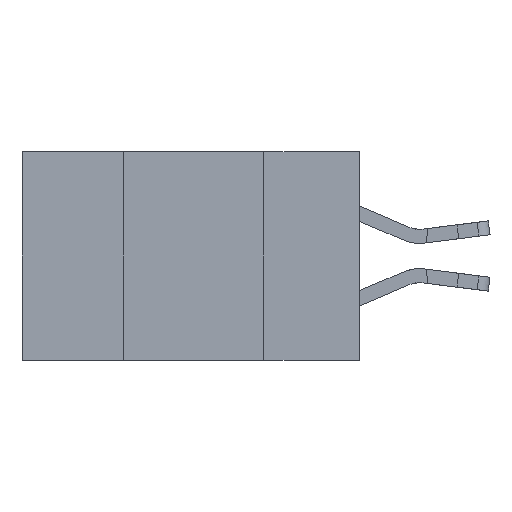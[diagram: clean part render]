
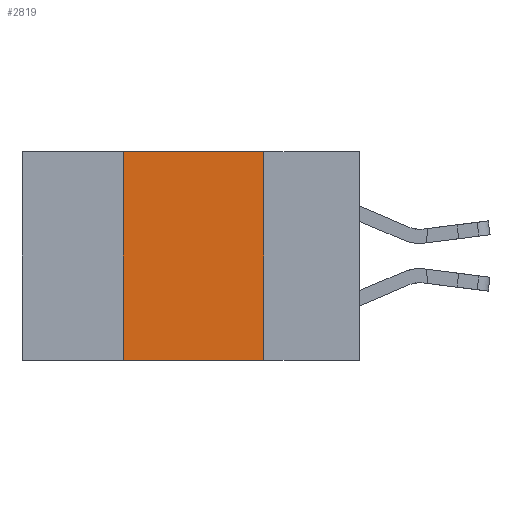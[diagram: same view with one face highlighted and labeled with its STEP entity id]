
A CAD part, left-side view. The second image highlights one B-rep face of the part: STEP entity #2819.
In plain terms, the highlighted planar face has unit normal (-1, 0, 0).
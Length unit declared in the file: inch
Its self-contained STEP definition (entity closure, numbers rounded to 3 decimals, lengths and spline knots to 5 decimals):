
#516 = VECTOR ( 'NONE', #9654, 39.37008 ) ;
#993 = VECTOR ( 'NONE', #11257, 39.37008 ) ;
#1025 = PLANE ( 'NONE',  #12570 ) ;
#1105 = DIRECTION ( 'NONE',  ( 0., 0., -1. ) ) ;
#2554 = DIRECTION ( 'NONE',  ( 0., 0., 1. ) ) ;
#2743 = CARTESIAN_POINT ( 'NONE',  ( 0., 0.42, -0.37 ) ) ;
#2819 = ADVANCED_FACE ( 'NONE', ( #15287 ), #1025, .F. ) ;
#4025 = EDGE_CURVE ( 'NONE', #15286, #12078, #6376, .T. ) ;
#4530 = ORIENTED_EDGE ( 'NONE', *, *, #14970, .F. ) ;
#4600 = VECTOR ( 'NONE', #2554, 39.37008 ) ;
#5540 = EDGE_CURVE ( 'NONE', #8309, #12078, #13459, .T. ) ;
#6212 = CARTESIAN_POINT ( 'NONE',  ( 0., 0.17, 0. ) ) ;
#6376 = LINE ( 'NONE', #6212, #993 ) ;
#6511 = DIRECTION ( 'NONE',  ( 1., 0., 0. ) ) ;
#6993 = CARTESIAN_POINT ( 'NONE',  ( 0., 0.42, 0. ) ) ;
#7165 = CARTESIAN_POINT ( 'NONE',  ( 0., 0.6, -0.37 ) ) ;
#8309 = VERTEX_POINT ( 'NONE', #2743 ) ;
#8828 = ORIENTED_EDGE ( 'NONE', *, *, #4025, .F. ) ;
#9654 = DIRECTION ( 'NONE',  ( 0., -1., 0. ) ) ;
#10044 = CARTESIAN_POINT ( 'NONE',  ( 0., 0.17, 0. ) ) ;
#10530 = ORIENTED_EDGE ( 'NONE', *, *, #15319, .F. ) ;
#11257 = DIRECTION ( 'NONE',  ( 0., 0., -1. ) ) ;
#11630 = VERTEX_POINT ( 'NONE', #6993 ) ;
#12078 = VERTEX_POINT ( 'NONE', #14674 ) ;
#12570 = AXIS2_PLACEMENT_3D ( 'NONE', #14137, #6511, #1105 ) ;
#12780 = VECTOR ( 'NONE', #14371, 39.37008 ) ;
#13029 = LINE ( 'NONE', #14219, #12780 ) ;
#13459 = LINE ( 'NONE', #7165, #516 ) ;
#14137 = CARTESIAN_POINT ( 'NONE',  ( 0., 0.6, 0. ) ) ;
#14219 = CARTESIAN_POINT ( 'NONE',  ( 0., 0.6, 0. ) ) ;
#14371 = DIRECTION ( 'NONE',  ( 0., -1., 0. ) ) ;
#14674 = CARTESIAN_POINT ( 'NONE',  ( 0., 0.17, -0.37 ) ) ;
#14970 = EDGE_CURVE ( 'NONE', #11630, #15286, #13029, .T. ) ;
#15069 = ORIENTED_EDGE ( 'NONE', *, *, #5540, .T. ) ;
#15268 = CARTESIAN_POINT ( 'NONE',  ( 0., 0.42, 0. ) ) ;
#15286 = VERTEX_POINT ( 'NONE', #10044 ) ;
#15287 = FACE_OUTER_BOUND ( 'NONE', #15519, .T. ) ;
#15319 = EDGE_CURVE ( 'NONE', #8309, #11630, #16235, .T. ) ;
#15519 = EDGE_LOOP ( 'NONE', ( #8828, #4530, #10530, #15069 ) ) ;
#16235 = LINE ( 'NONE', #15268, #4600 ) ;
